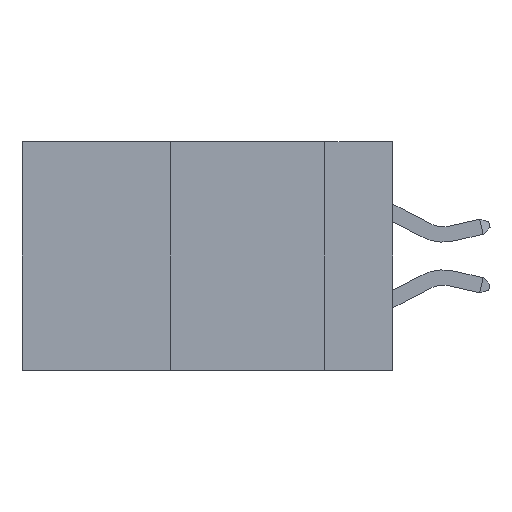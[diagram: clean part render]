
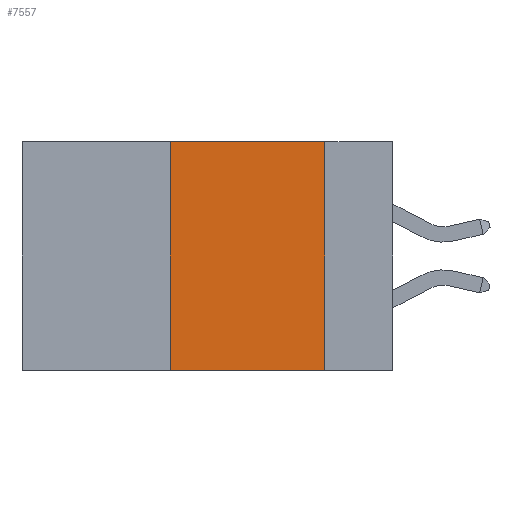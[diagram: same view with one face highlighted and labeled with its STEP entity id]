
A CAD part, left-side view. The second image highlights one B-rep face of the part: STEP entity #7557.
In plain terms, the highlighted planar face has unit normal (-1, 0, 0).
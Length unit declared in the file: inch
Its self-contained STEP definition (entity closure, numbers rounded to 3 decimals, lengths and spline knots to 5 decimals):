
#334 = VERTEX_POINT ( 'NONE', #23941 ) ;
#621 = EDGE_CURVE ( 'NONE', #19641, #334, #21201, .T. ) ;
#1585 = EDGE_CURVE ( 'NONE', #19641, #7060, #27375, .T. ) ;
#3131 = CARTESIAN_POINT ( 'NONE',  ( 0., 0.11, 0. ) ) ;
#4041 = ORIENTED_EDGE ( 'NONE', *, *, #621, .T. ) ;
#4461 = LINE ( 'NONE', #22485, #17427 ) ;
#5310 = VECTOR ( 'NONE', #26517, 39.37008 ) ;
#7060 = VERTEX_POINT ( 'NONE', #13537 ) ;
#7531 = CARTESIAN_POINT ( 'NONE',  ( 0., 0.6, -0.37 ) ) ;
#7557 = ADVANCED_FACE ( 'NONE', ( #16875 ), #22375, .F. ) ;
#8581 = VERTEX_POINT ( 'NONE', #3131 ) ;
#8694 = DIRECTION ( 'NONE',  ( 0., -1., 0. ) ) ;
#11718 = CARTESIAN_POINT ( 'NONE',  ( 0., 0.6, 0. ) ) ;
#12403 = ORIENTED_EDGE ( 'NONE', *, *, #1585, .F. ) ;
#13537 = CARTESIAN_POINT ( 'NONE',  ( 0., 0.36, 0. ) ) ;
#14183 = LINE ( 'NONE', #22174, #20156 ) ;
#16875 = FACE_OUTER_BOUND ( 'NONE', #31133, .T. ) ;
#17427 = VECTOR ( 'NONE', #32934, 39.37008 ) ;
#19294 = ORIENTED_EDGE ( 'NONE', *, *, #21978, .F. ) ;
#19641 = VERTEX_POINT ( 'NONE', #24486 ) ;
#20156 = VECTOR ( 'NONE', #8694, 39.37008 ) ;
#21201 = LINE ( 'NONE', #7531, #5310 ) ;
#21978 = EDGE_CURVE ( 'NONE', #7060, #8581, #14183, .T. ) ;
#22029 = DIRECTION ( 'NONE',  ( 1., 0., 0. ) ) ;
#22174 = CARTESIAN_POINT ( 'NONE',  ( 0., 0.6, 0. ) ) ;
#22375 = PLANE ( 'NONE',  #25056 ) ;
#22485 = CARTESIAN_POINT ( 'NONE',  ( 0., 0.11, 0. ) ) ;
#22549 = DIRECTION ( 'NONE',  ( 0., 0., -1. ) ) ;
#23671 = EDGE_CURVE ( 'NONE', #8581, #334, #4461, .T. ) ;
#23941 = CARTESIAN_POINT ( 'NONE',  ( 0., 0.11, -0.37 ) ) ;
#24486 = CARTESIAN_POINT ( 'NONE',  ( 0., 0.36, -0.37 ) ) ;
#25056 = AXIS2_PLACEMENT_3D ( 'NONE', #11718, #22029, #22549 ) ;
#26306 = VECTOR ( 'NONE', #32680, 39.37008 ) ;
#26517 = DIRECTION ( 'NONE',  ( 0., -1., 0. ) ) ;
#27375 = LINE ( 'NONE', #32149, #26306 ) ;
#27553 = ORIENTED_EDGE ( 'NONE', *, *, #23671, .F. ) ;
#31133 = EDGE_LOOP ( 'NONE', ( #27553, #19294, #12403, #4041 ) ) ;
#32149 = CARTESIAN_POINT ( 'NONE',  ( 0., 0.36, 0. ) ) ;
#32680 = DIRECTION ( 'NONE',  ( 0., 0., 1. ) ) ;
#32934 = DIRECTION ( 'NONE',  ( 0., 0., -1. ) ) ;
